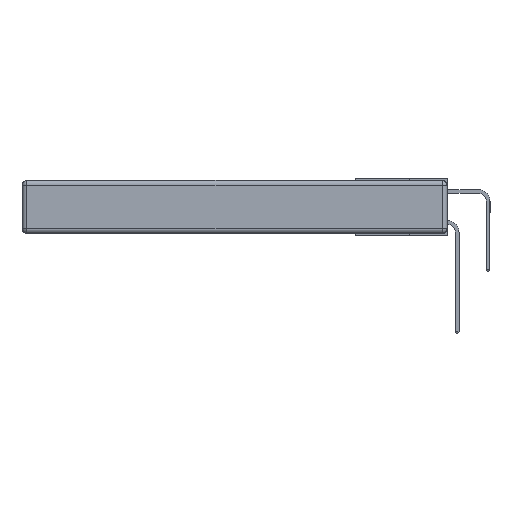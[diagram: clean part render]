
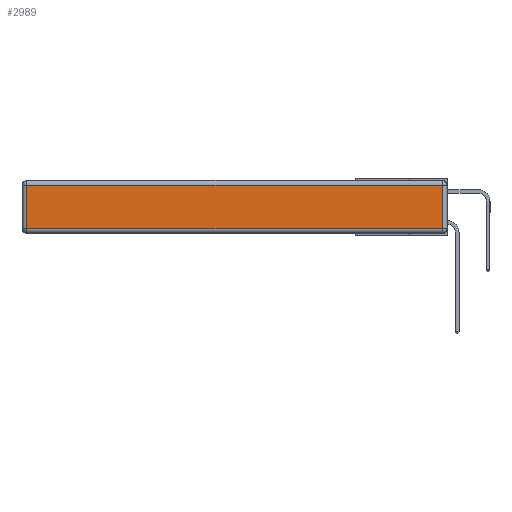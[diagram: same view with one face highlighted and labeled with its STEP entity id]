
A CAD part, left-side view. The second image highlights one B-rep face of the part: STEP entity #2989.
In plain terms, the highlighted planar face has unit normal (-1, 0, 0).
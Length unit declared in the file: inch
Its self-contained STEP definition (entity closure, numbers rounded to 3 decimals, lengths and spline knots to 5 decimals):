
#1489 = DIRECTION ( 'NONE',  ( 0., 1., 0. ) ) ;
#1670 = DIRECTION ( 'NONE',  ( 0., -1., 0. ) ) ;
#2989 = ADVANCED_FACE ( 'NONE', ( #5844 ), #26256, .T. ) ;
#4200 = VERTEX_POINT ( 'NONE', #21065 ) ;
#5701 = CARTESIAN_POINT ( 'NONE',  ( 0., 2.72, -0.343 ) ) ;
#5807 = DIRECTION ( 'NONE',  ( 0., 0., -1. ) ) ;
#5844 = FACE_OUTER_BOUND ( 'NONE', #22886, .T. ) ;
#7263 = AXIS2_PLACEMENT_3D ( 'NONE', #24459, #15370, #12968 ) ;
#10913 = VERTEX_POINT ( 'NONE', #15617 ) ;
#11129 = CARTESIAN_POINT ( 'NONE',  ( 0., 2.75, -0.03 ) ) ;
#12464 = LINE ( 'NONE', #5701, #16584 ) ;
#12492 = CARTESIAN_POINT ( 'NONE',  ( 0., 0.03, -0.03 ) ) ;
#12968 = DIRECTION ( 'NONE',  ( 0., 0., 1. ) ) ;
#13278 = LINE ( 'NONE', #16172, #23826 ) ;
#13307 = ORIENTED_EDGE ( 'NONE', *, *, #14045, .T. ) ;
#14045 = EDGE_CURVE ( 'NONE', #10913, #4200, #13278, .T. ) ;
#14100 = EDGE_CURVE ( 'NONE', #4200, #27833, #28385, .T. ) ;
#14261 = VECTOR ( 'NONE', #1489, 39.37008 ) ;
#15370 = DIRECTION ( 'NONE',  ( -1., 0., 0. ) ) ;
#15617 = CARTESIAN_POINT ( 'NONE',  ( 0., 2.72, -0.313 ) ) ;
#16172 = CARTESIAN_POINT ( 'NONE',  ( 0., 0., -0.313 ) ) ;
#16584 = VECTOR ( 'NONE', #5807, 39.37008 ) ;
#20339 = CARTESIAN_POINT ( 'NONE',  ( 0., 2.72, -0.03 ) ) ;
#20366 = ORIENTED_EDGE ( 'NONE', *, *, #14100, .T. ) ;
#21065 = CARTESIAN_POINT ( 'NONE',  ( 0., 0.03, -0.313 ) ) ;
#21398 = DIRECTION ( 'NONE',  ( 0., 0., 1. ) ) ;
#21935 = VECTOR ( 'NONE', #21398, 39.37008 ) ;
#22068 = EDGE_CURVE ( 'NONE', #26995, #10913, #12464, .T. ) ;
#22886 = EDGE_LOOP ( 'NONE', ( #13307, #20366, #28405, #29554 ) ) ;
#23826 = VECTOR ( 'NONE', #1670, 39.37008 ) ;
#24459 = CARTESIAN_POINT ( 'NONE',  ( 0., 0., -0.343 ) ) ;
#26144 = EDGE_CURVE ( 'NONE', #27833, #26995, #30879, .T. ) ;
#26256 = PLANE ( 'NONE',  #7263 ) ;
#26995 = VERTEX_POINT ( 'NONE', #20339 ) ;
#27833 = VERTEX_POINT ( 'NONE', #12492 ) ;
#28385 = LINE ( 'NONE', #30860, #21935 ) ;
#28405 = ORIENTED_EDGE ( 'NONE', *, *, #26144, .T. ) ;
#29554 = ORIENTED_EDGE ( 'NONE', *, *, #22068, .T. ) ;
#30860 = CARTESIAN_POINT ( 'NONE',  ( 0., 0.03, -0.343 ) ) ;
#30879 = LINE ( 'NONE', #11129, #14261 ) ;
